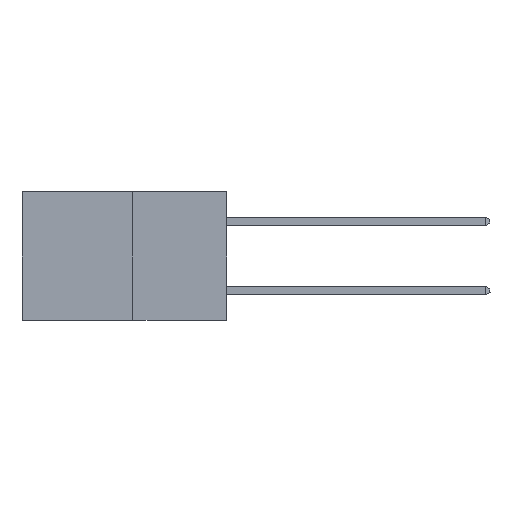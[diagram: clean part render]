
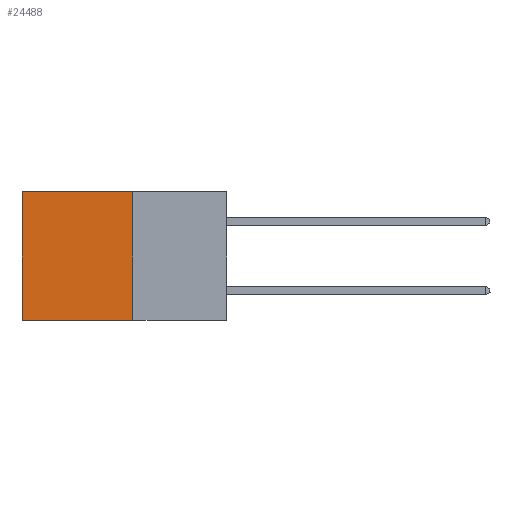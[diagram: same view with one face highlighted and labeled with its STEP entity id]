
A CAD part, left-side view. The second image highlights one B-rep face of the part: STEP entity #24488.
In plain terms, the highlighted planar face has unit normal (-1, 0, 0).
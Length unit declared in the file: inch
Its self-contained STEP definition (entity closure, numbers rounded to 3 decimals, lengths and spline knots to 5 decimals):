
#2578 = EDGE_CURVE ( 'NONE', #14825, #18880, #28737, .T. ) ;
#3513 = CARTESIAN_POINT ( 'NONE',  ( 0.277, 0.27, -0.37 ) ) ;
#4539 = VECTOR ( 'NONE', #23654, 39.37008 ) ;
#6376 = CARTESIAN_POINT ( 'NONE',  ( 0.277, 0.27, -0.37 ) ) ;
#7950 = CARTESIAN_POINT ( 'NONE',  ( 0.277, 0.59, -0.37 ) ) ;
#8699 = AXIS2_PLACEMENT_3D ( 'NONE', #20908, #23101, #9693 ) ;
#9224 = VERTEX_POINT ( 'NONE', #17229 ) ;
#9693 = DIRECTION ( 'NONE',  ( 0., 0., -1. ) ) ;
#9915 = LINE ( 'NONE', #7950, #4539 ) ;
#10044 = LINE ( 'NONE', #3513, #27175 ) ;
#10980 = LINE ( 'NONE', #26002, #16286 ) ;
#11926 = VERTEX_POINT ( 'NONE', #23951 ) ;
#12573 = DIRECTION ( 'NONE',  ( 0., 1., 0. ) ) ;
#14825 = VERTEX_POINT ( 'NONE', #6376 ) ;
#15830 = FACE_OUTER_BOUND ( 'NONE', #21251, .T. ) ;
#16286 = VECTOR ( 'NONE', #12573, 39.37008 ) ;
#17229 = CARTESIAN_POINT ( 'NONE',  ( 0.277, 0.59, 0. ) ) ;
#17253 = DIRECTION ( 'NONE',  ( 0., 0., -1. ) ) ;
#17619 = EDGE_CURVE ( 'NONE', #11926, #9224, #10980, .T. ) ;
#18668 = PLANE ( 'NONE',  #8699 ) ;
#18880 = VERTEX_POINT ( 'NONE', #21485 ) ;
#19199 = ORIENTED_EDGE ( 'NONE', *, *, #28862, .T. ) ;
#20908 = CARTESIAN_POINT ( 'NONE',  ( 0.277, 0.27, -0.37 ) ) ;
#21251 = EDGE_LOOP ( 'NONE', ( #19199, #28857, #26427, #28023 ) ) ;
#21485 = CARTESIAN_POINT ( 'NONE',  ( 0.277, 0.59, -0.37 ) ) ;
#23101 = DIRECTION ( 'NONE',  ( 1., 0., 0. ) ) ;
#23654 = DIRECTION ( 'NONE',  ( 0., 0., -1. ) ) ;
#23951 = CARTESIAN_POINT ( 'NONE',  ( 0.277, 0.27, 0. ) ) ;
#24488 = ADVANCED_FACE ( 'NONE', ( #15830 ), #18668, .F. ) ;
#26002 = CARTESIAN_POINT ( 'NONE',  ( 0.277, 0.27, 0. ) ) ;
#26011 = EDGE_CURVE ( 'NONE', #11926, #14825, #10044, .T. ) ;
#26406 = CARTESIAN_POINT ( 'NONE',  ( 0.277, 0.27, -0.37 ) ) ;
#26427 = ORIENTED_EDGE ( 'NONE', *, *, #26011, .F. ) ;
#26510 = DIRECTION ( 'NONE',  ( 0., 1., 0. ) ) ;
#27175 = VECTOR ( 'NONE', #17253, 39.37008 ) ;
#28023 = ORIENTED_EDGE ( 'NONE', *, *, #17619, .T. ) ;
#28052 = VECTOR ( 'NONE', #26510, 39.37008 ) ;
#28737 = LINE ( 'NONE', #26406, #28052 ) ;
#28857 = ORIENTED_EDGE ( 'NONE', *, *, #2578, .F. ) ;
#28862 = EDGE_CURVE ( 'NONE', #9224, #18880, #9915, .T. ) ;
